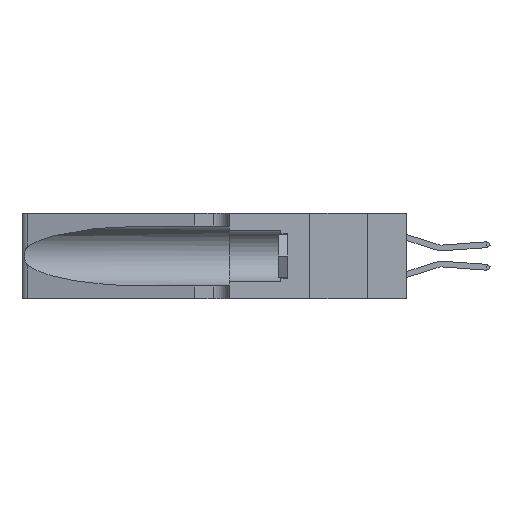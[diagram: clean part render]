
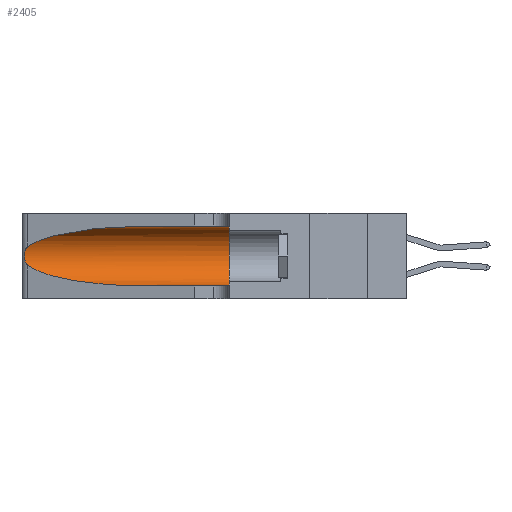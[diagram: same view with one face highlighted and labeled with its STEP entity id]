
A CAD part, left-side view. The second image highlights one B-rep face of the part: STEP entity #2405.
In plain terms, the highlighted cylindrical face has radius 3.308 mm (diameter 6.617 mm), a partial arc.
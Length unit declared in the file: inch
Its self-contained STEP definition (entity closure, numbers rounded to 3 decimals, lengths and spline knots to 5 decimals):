
#290 = CARTESIAN_POINT ( 'NONE',  ( 0.1305, 1.61858, 0.185 ) ) ;
#770 = CARTESIAN_POINT ( 'NONE',  ( 0.1305, 0.35, 0.31525 ) ) ;
#1219 = CARTESIAN_POINT ( 'NONE',  ( 0.1305, 0.72297, 0.05475 ) ) ;
#1363 = ORIENTED_EDGE ( 'NONE', *, *, #8183, .F. ) ;
#1636 = CARTESIAN_POINT ( 'NONE',  ( 0.26075, 1.23896, 0.19203 ) ) ;
#1851 = CARTESIAN_POINT ( 'NONE',  ( 0.25555, 1.22994, 0.2215 ) ) ;
#2337 = VERTEX_POINT ( 'NONE', #3310 ) ;
#2405 = ADVANCED_FACE ( 'NONE', ( #7175 ), #13560, .F. ) ;
#2428 =( BOUNDED_CURVE ( )  B_SPLINE_CURVE ( 3, ( #20446, #18887, #11823, #1219 ),
 .UNSPECIFIED., .F., .T. ) 
 B_SPLINE_CURVE_WITH_KNOTS ( ( 4, 4 ),
 ( 3.44316, 4.71239 ),
 .UNSPECIFIED. ) 
 CURVE ( )  GEOMETRIC_REPRESENTATION_ITEM ( )  RATIONAL_B_SPLINE_CURVE ( ( 1., 0.87, 0.87, 1. ) ) 
 REPRESENTATION_ITEM ( '' )  );
#2551 = VECTOR ( 'NONE', #8569, 39.37008 ) ;
#2626 = ORIENTED_EDGE ( 'NONE', *, *, #22875, .T. ) ;
#3310 = CARTESIAN_POINT ( 'NONE',  ( 0.1305, 0.72297, 0.31525 ) ) ;
#3477 = CARTESIAN_POINT ( 'NONE',  ( 0.26018, 1.23835, 0.19895 ) ) ;
#5130 = CARTESIAN_POINT ( 'NONE',  ( 0.25854, 1.2359, 0.20912 ) ) ;
#5210 = CARTESIAN_POINT ( 'NONE',  ( 0.25555, 1.22993, 0.14849 ) ) ;
#5356 = CARTESIAN_POINT ( 'NONE',  ( 0.25789, 1.23486, 0.15765 ) ) ;
#6043 = DIRECTION ( 'NONE',  ( 0., 0., 1. ) ) ;
#6591 = CARTESIAN_POINT ( 'NONE',  ( 0.1305, 0.72297, 0.05475 ) ) ;
#7175 = FACE_OUTER_BOUND ( 'NONE', #11031, .T. ) ;
#7453 = DIRECTION ( 'NONE',  ( 0., -1., 0. ) ) ;
#8077 = CARTESIAN_POINT ( 'NONE',  ( 0.2373, 1.15595, 0.28018 ) ) ;
#8183 = EDGE_CURVE ( 'NONE', #2337, #17153, #16695, .T. ) ;
#8452 = ORIENTED_EDGE ( 'NONE', *, *, #15146, .T. ) ;
#8569 = DIRECTION ( 'NONE',  ( 0., -1., 0. ) ) ;
#8809 = AXIS2_PLACEMENT_3D ( 'NONE', #290, #7453, #19657 ) ;
#8838 = CARTESIAN_POINT ( 'NONE',  ( 0.25639, 1.23186, 0.15144 ) ) ;
#9362 = EDGE_CURVE ( 'NONE', #14153, #19540, #22777, .T. ) ;
#9617 = ORIENTED_EDGE ( 'NONE', *, *, #22116, .T. ) ;
#10186 = AXIS2_PLACEMENT_3D ( 'NONE', #16645, #13134, #6043 ) ;
#10386 = EDGE_CURVE ( 'NONE', #17153, #16330, #14739, .T. ) ;
#11031 = EDGE_LOOP ( 'NONE', ( #9617, #14185, #2626, #8452, #20351, #1363 ) ) ;
#11823 = CARTESIAN_POINT ( 'NONE',  ( 0.18966, 0.96281, 0.05475 ) ) ;
#12233 = CARTESIAN_POINT ( 'NONE',  ( 0.26075, 1.23896, 0.178 ) ) ;
#12302 = CARTESIAN_POINT ( 'NONE',  ( 0.26017, 1.23833, 0.17102 ) ) ;
#12521 = CARTESIAN_POINT ( 'NONE',  ( 0.25487, 1.22718, 0.22369 ) ) ;
#12815 = VERTEX_POINT ( 'NONE', #6591 ) ;
#13134 = DIRECTION ( 'NONE',  ( 0., 1., 0. ) ) ;
#13560 = CYLINDRICAL_SURFACE ( 'NONE', #8809, 0.13025 ) ;
#14153 = VERTEX_POINT ( 'NONE', #16414 ) ;
#14185 = ORIENTED_EDGE ( 'NONE', *, *, #9362, .T. ) ;
#14230 = CARTESIAN_POINT ( 'NONE',  ( 0.25856, 1.23593, 0.16098 ) ) ;
#14739 = CIRCLE ( 'NONE', #10186, 0.13025 ) ;
#15124 = CARTESIAN_POINT ( 'NONE',  ( 0.18966, 0.96281, 0.31525 ) ) ;
#15146 = EDGE_CURVE ( 'NONE', #12815, #16330, #19996, .T. ) ;
#15758 = CARTESIAN_POINT ( 'NONE',  ( 0.25639, 1.23184, 0.21858 ) ) ;
#16330 = VERTEX_POINT ( 'NONE', #21471 ) ;
#16414 = CARTESIAN_POINT ( 'NONE',  ( 0.25487, 1.22718, 0.22369 ) ) ;
#16645 = CARTESIAN_POINT ( 'NONE',  ( 0.1305, 0.35, 0.185 ) ) ;
#16695 = LINE ( 'NONE', #19166, #2551 ) ;
#16984 = VECTOR ( 'NONE', #20767, 39.37008 ) ;
#17153 = VERTEX_POINT ( 'NONE', #770 ) ;
#17532 = CARTESIAN_POINT ( 'NONE',  ( 0.25487, 1.22718, 0.14631 ) ) ;
#17749 = CARTESIAN_POINT ( 'NONE',  ( 0.25787, 1.23484, 0.2124 ) ) ;
#18600 = CARTESIAN_POINT ( 'NONE',  ( 0.1305, 0.72297, 0.31525 ) ) ;
#18887 = CARTESIAN_POINT ( 'NONE',  ( 0.2373, 1.15595, 0.08982 ) ) ;
#19011 = CARTESIAN_POINT ( 'NONE',  ( 0.1305, 1.61858, 0.05475 ) ) ;
#19166 = CARTESIAN_POINT ( 'NONE',  ( 0.1305, 1.61858, 0.31525 ) ) ;
#19540 = VERTEX_POINT ( 'NONE', #20869 ) ;
#19657 = DIRECTION ( 'NONE',  ( 0., 0., -1. ) ) ;
#19996 = LINE ( 'NONE', #19011, #16984 ) ;
#20351 = ORIENTED_EDGE ( 'NONE', *, *, #10386, .F. ) ;
#20446 = CARTESIAN_POINT ( 'NONE',  ( 0.25487, 1.22718, 0.14631 ) ) ;
#20767 = DIRECTION ( 'NONE',  ( 0., -1., 0. ) ) ;
#20869 = CARTESIAN_POINT ( 'NONE',  ( 0.25487, 1.22718, 0.14631 ) ) ;
#21471 = CARTESIAN_POINT ( 'NONE',  ( 0.1305, 0.35, 0.05475 ) ) ;
#21720 =( BOUNDED_CURVE ( )  B_SPLINE_CURVE ( 3, ( #18600, #15124, #8077, #22408 ),
 .UNSPECIFIED., .F., .F. ) 
 B_SPLINE_CURVE_WITH_KNOTS ( ( 4, 4 ),
 ( 1.5708, 2.84003 ),
 .UNSPECIFIED. ) 
 CURVE ( )  GEOMETRIC_REPRESENTATION_ITEM ( )  RATIONAL_B_SPLINE_CURVE ( ( 1., 0.87, 0.87, 1. ) ) 
 REPRESENTATION_ITEM ( '' )  );
#22116 = EDGE_CURVE ( 'NONE', #2337, #14153, #21720, .T. ) ;
#22408 = CARTESIAN_POINT ( 'NONE',  ( 0.25487, 1.22718, 0.22369 ) ) ;
#22777 = B_SPLINE_CURVE_WITH_KNOTS ( 'NONE', 3,
 ( #12521, #1851, #15758, #17749, #5130, #3477, #1636, #12233, #12302, #14230, #5356, #8838, #5210, #17532 ),
 .UNSPECIFIED., .F., .F.,
 ( 4, 2, 2, 2, 2, 2, 4 ),
 ( 0., 0.00027, 0.00053, 0.00107, 0.0016, 0.00187, 0.00214 ),
 .UNSPECIFIED. ) ;
#22875 = EDGE_CURVE ( 'NONE', #19540, #12815, #2428, .T. ) ;
